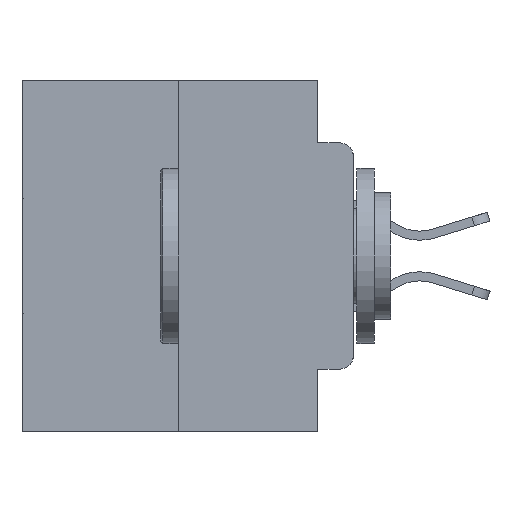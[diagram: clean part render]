
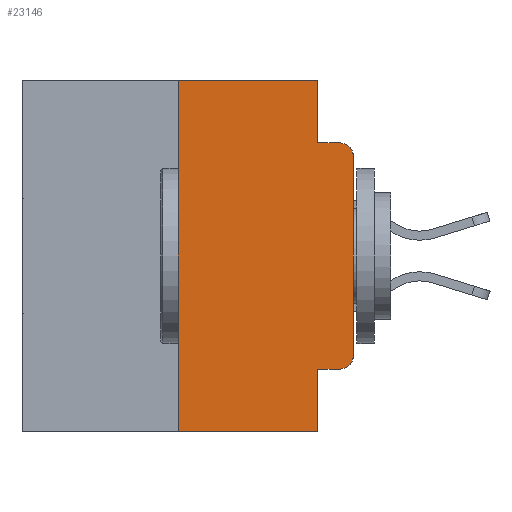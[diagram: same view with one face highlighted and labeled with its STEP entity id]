
A CAD part, left-side view. The second image highlights one B-rep face of the part: STEP entity #23146.
In plain terms, the highlighted planar face has unit normal (-1, 0, 0).
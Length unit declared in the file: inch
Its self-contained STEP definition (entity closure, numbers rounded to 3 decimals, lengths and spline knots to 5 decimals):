
#67 = VECTOR ( 'NONE', #5352, 39.37008 ) ;
#501 = FACE_OUTER_BOUND ( 'NONE', #9594, .T. ) ;
#562 = VERTEX_POINT ( 'NONE', #8065 ) ;
#850 = CARTESIAN_POINT ( 'NONE',  ( 0., 0.25, 0. ) ) ;
#920 = LINE ( 'NONE', #9601, #21899 ) ;
#1715 = DIRECTION ( 'NONE',  ( 0., 0., -1. ) ) ;
#2035 = CARTESIAN_POINT ( 'NONE',  ( 0., 0.02, -0.1085 ) ) ;
#2398 = DIRECTION ( 'NONE',  ( 0., -1., 0. ) ) ;
#2930 = CARTESIAN_POINT ( 'NONE',  ( 0., 0.25, -0.5 ) ) ;
#3074 = VERTEX_POINT ( 'NONE', #2930 ) ;
#3470 = EDGE_CURVE ( 'NONE', #3074, #18677, #16342, .T. ) ;
#3660 = CARTESIAN_POINT ( 'NONE',  ( 0., 0.051, -0.4115 ) ) ;
#3661 = DIRECTION ( 'NONE',  ( 0., -1., 0. ) ) ;
#5059 = VERTEX_POINT ( 'NONE', #3660 ) ;
#5151 = AXIS2_PLACEMENT_3D ( 'NONE', #17783, #26589, #1715 ) ;
#5299 = ORIENTED_EDGE ( 'NONE', *, *, #19315, .T. ) ;
#5312 = CIRCLE ( 'NONE', #23315, 0.02 ) ;
#5352 = DIRECTION ( 'NONE',  ( 0., 0., 1. ) ) ;
#5939 = LINE ( 'NONE', #8395, #21720 ) ;
#6816 = EDGE_CURVE ( 'NONE', #20285, #23598, #5312, .T. ) ;
#7320 = ORIENTED_EDGE ( 'NONE', *, *, #14923, .F. ) ;
#7399 = VERTEX_POINT ( 'NONE', #12059 ) ;
#8065 = CARTESIAN_POINT ( 'NONE',  ( 0., 0.051, -0.0885 ) ) ;
#8277 = EDGE_CURVE ( 'NONE', #18677, #16031, #23821, .T. ) ;
#8395 = CARTESIAN_POINT ( 'NONE',  ( 0., 0.051, -0.0885 ) ) ;
#8489 = DIRECTION ( 'NONE',  ( 0., -1., 0. ) ) ;
#8576 = ORIENTED_EDGE ( 'NONE', *, *, #9806, .T. ) ;
#9496 = ORIENTED_EDGE ( 'NONE', *, *, #6816, .T. ) ;
#9594 = EDGE_LOOP ( 'NONE', ( #19905, #9496, #15475, #23014, #20848, #17035, #23637, #7320, #5299, #8576 ) ) ;
#9601 = CARTESIAN_POINT ( 'NONE',  ( 0., 0.473, -0.5 ) ) ;
#9806 = EDGE_CURVE ( 'NONE', #24716, #23445, #21323, .T. ) ;
#10275 = CARTESIAN_POINT ( 'NONE',  ( 0., 0.051, 0. ) ) ;
#10550 = LINE ( 'NONE', #19376, #19117 ) ;
#11062 = CARTESIAN_POINT ( 'NONE',  ( 0., 0.051, -0.4115 ) ) ;
#11214 = AXIS2_PLACEMENT_3D ( 'NONE', #17901, #11364, #24669 ) ;
#11364 = DIRECTION ( 'NONE',  ( 1., 0., 0. ) ) ;
#11564 = CARTESIAN_POINT ( 'NONE',  ( 0., 0., -0.1085 ) ) ;
#11647 = PLANE ( 'NONE',  #11214 ) ;
#12059 = CARTESIAN_POINT ( 'NONE',  ( 0., 0.051, -0.5 ) ) ;
#13042 = CARTESIAN_POINT ( 'NONE',  ( 0., 0.051, 0. ) ) ;
#13111 = LINE ( 'NONE', #11062, #15250 ) ;
#14025 = EDGE_CURVE ( 'NONE', #3074, #7399, #920, .T. ) ;
#14620 = EDGE_CURVE ( 'NONE', #16031, #562, #26180, .T. ) ;
#14923 = EDGE_CURVE ( 'NONE', #5059, #7399, #25009, .T. ) ;
#15202 = DIRECTION ( 'NONE',  ( 0., 0., -1. ) ) ;
#15250 = VECTOR ( 'NONE', #2398, 39.37008 ) ;
#15475 = ORIENTED_EDGE ( 'NONE', *, *, #19022, .F. ) ;
#16031 = VERTEX_POINT ( 'NONE', #13042 ) ;
#16342 = LINE ( 'NONE', #850, #67 ) ;
#17035 = ORIENTED_EDGE ( 'NONE', *, *, #3470, .F. ) ;
#17232 = DIRECTION ( 'NONE',  ( -1., 0., 0. ) ) ;
#17783 = CARTESIAN_POINT ( 'NONE',  ( 0., 0.02, -0.3915 ) ) ;
#17901 = CARTESIAN_POINT ( 'NONE',  ( 0., 0.473, 0. ) ) ;
#18677 = VERTEX_POINT ( 'NONE', #23759 ) ;
#18794 = CARTESIAN_POINT ( 'NONE',  ( 0., 0.051, 0. ) ) ;
#18957 = DIRECTION ( 'NONE',  ( 0., 0., 1. ) ) ;
#19022 = EDGE_CURVE ( 'NONE', #562, #23598, #5939, .T. ) ;
#19117 = VECTOR ( 'NONE', #18957, 39.37008 ) ;
#19315 = EDGE_CURVE ( 'NONE', #5059, #24716, #13111, .T. ) ;
#19376 = CARTESIAN_POINT ( 'NONE',  ( 0., 0., 0. ) ) ;
#19683 = DIRECTION ( 'NONE',  ( 0., -1., 0. ) ) ;
#19686 = DIRECTION ( 'NONE',  ( 0., 0., -1. ) ) ;
#19905 = ORIENTED_EDGE ( 'NONE', *, *, #25494, .T. ) ;
#20285 = VERTEX_POINT ( 'NONE', #11564 ) ;
#20540 = VECTOR ( 'NONE', #15202, 39.37008 ) ;
#20794 = VECTOR ( 'NONE', #8489, 39.37008 ) ;
#20848 = ORIENTED_EDGE ( 'NONE', *, *, #8277, .F. ) ;
#21323 = CIRCLE ( 'NONE', #5151, 0.02 ) ;
#21617 = CARTESIAN_POINT ( 'NONE',  ( 0., 0.02, -0.0885 ) ) ;
#21720 = VECTOR ( 'NONE', #19683, 39.37008 ) ;
#21899 = VECTOR ( 'NONE', #3661, 39.37008 ) ;
#22847 = CARTESIAN_POINT ( 'NONE',  ( 0., 0.02, -0.4115 ) ) ;
#23014 = ORIENTED_EDGE ( 'NONE', *, *, #14620, .F. ) ;
#23146 = ADVANCED_FACE ( 'NONE', ( #501 ), #11647, .F. ) ;
#23315 = AXIS2_PLACEMENT_3D ( 'NONE', #2035, #17232, #19686 ) ;
#23445 = VERTEX_POINT ( 'NONE', #23492 ) ;
#23492 = CARTESIAN_POINT ( 'NONE',  ( 0., 0., -0.3915 ) ) ;
#23598 = VERTEX_POINT ( 'NONE', #21617 ) ;
#23637 = ORIENTED_EDGE ( 'NONE', *, *, #14025, .T. ) ;
#23759 = CARTESIAN_POINT ( 'NONE',  ( 0., 0.25, 0. ) ) ;
#23821 = LINE ( 'NONE', #25995, #20794 ) ;
#24669 = DIRECTION ( 'NONE',  ( 0., 0., -1. ) ) ;
#24716 = VERTEX_POINT ( 'NONE', #22847 ) ;
#25009 = LINE ( 'NONE', #18794, #26086 ) ;
#25494 = EDGE_CURVE ( 'NONE', #23445, #20285, #10550, .T. ) ;
#25995 = CARTESIAN_POINT ( 'NONE',  ( 0., 0.473, 0. ) ) ;
#26086 = VECTOR ( 'NONE', #27169, 39.37008 ) ;
#26180 = LINE ( 'NONE', #10275, #20540 ) ;
#26589 = DIRECTION ( 'NONE',  ( -1., 0., 0. ) ) ;
#27169 = DIRECTION ( 'NONE',  ( 0., 0., -1. ) ) ;
